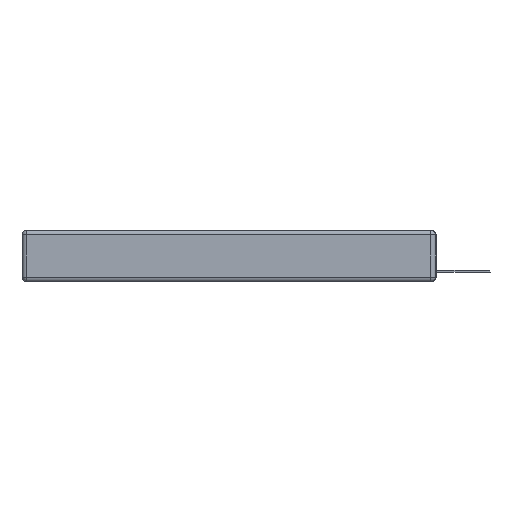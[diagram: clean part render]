
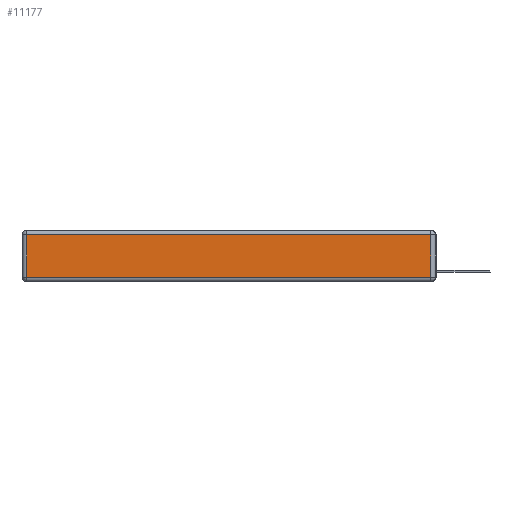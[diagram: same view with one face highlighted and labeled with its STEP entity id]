
A CAD part, left-side view. The second image highlights one B-rep face of the part: STEP entity #11177.
In plain terms, the highlighted planar face has unit normal (-1, 0, 0).
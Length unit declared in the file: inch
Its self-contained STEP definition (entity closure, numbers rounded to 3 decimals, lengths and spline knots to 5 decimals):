
#1031 = FACE_OUTER_BOUND ( 'NONE', #3103, .T. ) ;
#1078 = CARTESIAN_POINT ( 'NONE',  ( 0., 0.03, -0.03 ) ) ;
#1712 = ORIENTED_EDGE ( 'NONE', *, *, #17356, .T. ) ;
#2630 = CARTESIAN_POINT ( 'NONE',  ( 0., 2.72, -0.03 ) ) ;
#2858 = CARTESIAN_POINT ( 'NONE',  ( 0., 2.75, -0.03 ) ) ;
#3103 = EDGE_LOOP ( 'NONE', ( #22404, #3882, #20698, #1712 ) ) ;
#3633 = LINE ( 'NONE', #2858, #7374 ) ;
#3882 = ORIENTED_EDGE ( 'NONE', *, *, #21693, .T. ) ;
#3930 = VECTOR ( 'NONE', #13823, 39.37008 ) ;
#4273 = CARTESIAN_POINT ( 'NONE',  ( 0., 0., -0.313 ) ) ;
#5882 = LINE ( 'NONE', #20675, #21021 ) ;
#6941 = PLANE ( 'NONE',  #12230 ) ;
#7374 = VECTOR ( 'NONE', #14185, 39.37008 ) ;
#8347 = VECTOR ( 'NONE', #15372, 39.37008 ) ;
#10345 = CARTESIAN_POINT ( 'NONE',  ( 0., 2.72, -0.313 ) ) ;
#10559 = VERTEX_POINT ( 'NONE', #2630 ) ;
#11177 = ADVANCED_FACE ( 'NONE', ( #1031 ), #6941, .T. ) ;
#11427 = DIRECTION ( 'NONE',  ( 0., 0., 1. ) ) ;
#12230 = AXIS2_PLACEMENT_3D ( 'NONE', #21502, #17860, #23373 ) ;
#13539 = VERTEX_POINT ( 'NONE', #1078 ) ;
#13668 = CARTESIAN_POINT ( 'NONE',  ( 0., 0.03, -0.313 ) ) ;
#13677 = CARTESIAN_POINT ( 'NONE',  ( 0., 2.72, -0.343 ) ) ;
#13782 = VERTEX_POINT ( 'NONE', #13668 ) ;
#13823 = DIRECTION ( 'NONE',  ( 0., -1., 0. ) ) ;
#13865 = LINE ( 'NONE', #4273, #3930 ) ;
#14185 = DIRECTION ( 'NONE',  ( 0., 1., 0. ) ) ;
#15372 = DIRECTION ( 'NONE',  ( 0., 0., -1. ) ) ;
#17356 = EDGE_CURVE ( 'NONE', #10559, #22427, #17958, .T. ) ;
#17860 = DIRECTION ( 'NONE',  ( -1., 0., 0. ) ) ;
#17958 = LINE ( 'NONE', #13677, #8347 ) ;
#18038 = EDGE_CURVE ( 'NONE', #22427, #13782, #13865, .T. ) ;
#20675 = CARTESIAN_POINT ( 'NONE',  ( 0., 0.03, -0.343 ) ) ;
#20698 = ORIENTED_EDGE ( 'NONE', *, *, #21256, .T. ) ;
#21021 = VECTOR ( 'NONE', #11427, 39.37008 ) ;
#21256 = EDGE_CURVE ( 'NONE', #13539, #10559, #3633, .T. ) ;
#21502 = CARTESIAN_POINT ( 'NONE',  ( 0., 0., -0.343 ) ) ;
#21693 = EDGE_CURVE ( 'NONE', #13782, #13539, #5882, .T. ) ;
#22404 = ORIENTED_EDGE ( 'NONE', *, *, #18038, .T. ) ;
#22427 = VERTEX_POINT ( 'NONE', #10345 ) ;
#23373 = DIRECTION ( 'NONE',  ( 0., 0., 1. ) ) ;
